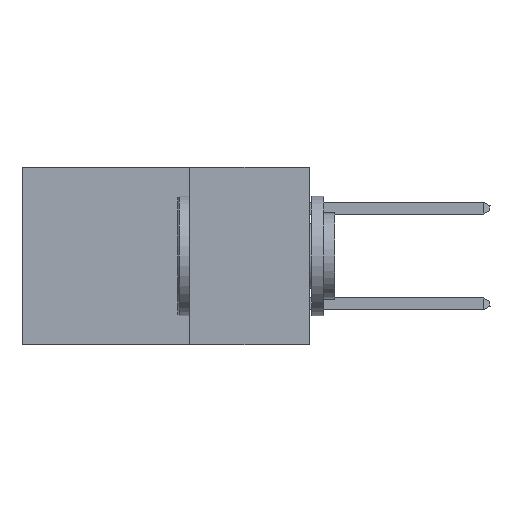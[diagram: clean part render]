
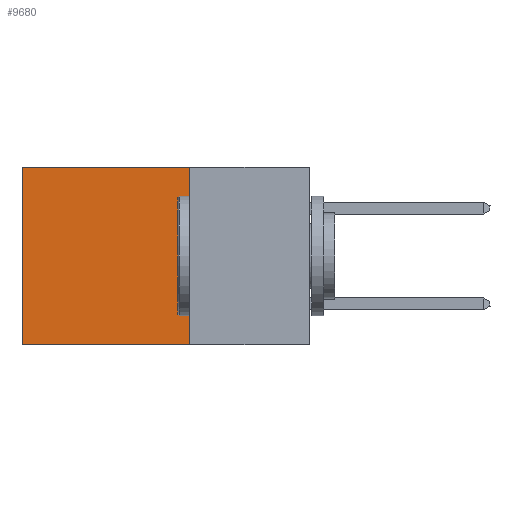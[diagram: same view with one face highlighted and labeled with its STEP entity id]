
A CAD part, left-side view. The second image highlights one B-rep face of the part: STEP entity #9680.
In plain terms, the highlighted planar face has unit normal (-1, 0, 0).
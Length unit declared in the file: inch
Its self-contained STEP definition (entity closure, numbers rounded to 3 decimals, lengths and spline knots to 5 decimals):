
#681 = DIRECTION ( 'NONE',  ( 0., 0., -1. ) ) ;
#1532 = EDGE_LOOP ( 'NONE', ( #10263, #7408, #1742, #7679 ) ) ;
#1534 = VECTOR ( 'NONE', #5011, 39.37008 ) ;
#1540 = VECTOR ( 'NONE', #8751, 39.37008 ) ;
#1742 = ORIENTED_EDGE ( 'NONE', *, *, #8023, .F. ) ;
#1813 = AXIS2_PLACEMENT_3D ( 'NONE', #2339, #5754, #681 ) ;
#1914 = CARTESIAN_POINT ( 'NONE',  ( 0.2875, 0.25, -0.37 ) ) ;
#2339 = CARTESIAN_POINT ( 'NONE',  ( 0.2875, 0.25, 0. ) ) ;
#2907 = CARTESIAN_POINT ( 'NONE',  ( 0.2875, 0.6, 0. ) ) ;
#3188 = PLANE ( 'NONE',  #1813 ) ;
#3259 = VECTOR ( 'NONE', #3657, 39.37008 ) ;
#3532 = LINE ( 'NONE', #2907, #1540 ) ;
#3657 = DIRECTION ( 'NONE',  ( 0., 1., 0. ) ) ;
#3785 = LINE ( 'NONE', #10820, #1534 ) ;
#4474 = VERTEX_POINT ( 'NONE', #10318 ) ;
#4600 = VERTEX_POINT ( 'NONE', #7164 ) ;
#4610 = CARTESIAN_POINT ( 'NONE',  ( 0.2875, 0.25, 0. ) ) ;
#5011 = DIRECTION ( 'NONE',  ( 0., 1., 0. ) ) ;
#5233 = VERTEX_POINT ( 'NONE', #7151 ) ;
#5248 = LINE ( 'NONE', #9457, #3259 ) ;
#5555 = LINE ( 'NONE', #4610, #7756 ) ;
#5754 = DIRECTION ( 'NONE',  ( 1., 0., 0. ) ) ;
#7151 = CARTESIAN_POINT ( 'NONE',  ( 0.2875, 0.25, 0. ) ) ;
#7164 = CARTESIAN_POINT ( 'NONE',  ( 0.2875, 0.6, -0.37 ) ) ;
#7372 = VERTEX_POINT ( 'NONE', #1914 ) ;
#7408 = ORIENTED_EDGE ( 'NONE', *, *, #9362, .F. ) ;
#7679 = ORIENTED_EDGE ( 'NONE', *, *, #9761, .T. ) ;
#7756 = VECTOR ( 'NONE', #8737, 39.37008 ) ;
#8023 = EDGE_CURVE ( 'NONE', #5233, #7372, #5555, .T. ) ;
#8731 = FACE_OUTER_BOUND ( 'NONE', #1532, .T. ) ;
#8737 = DIRECTION ( 'NONE',  ( 0., 0., -1. ) ) ;
#8751 = DIRECTION ( 'NONE',  ( 0., 0., -1. ) ) ;
#9362 = EDGE_CURVE ( 'NONE', #7372, #4600, #5248, .T. ) ;
#9457 = CARTESIAN_POINT ( 'NONE',  ( 0.2875, 0.25, -0.37 ) ) ;
#9680 = ADVANCED_FACE ( 'NONE', ( #8731 ), #3188, .F. ) ;
#9761 = EDGE_CURVE ( 'NONE', #5233, #4474, #3785, .T. ) ;
#10263 = ORIENTED_EDGE ( 'NONE', *, *, #10796, .T. ) ;
#10318 = CARTESIAN_POINT ( 'NONE',  ( 0.2875, 0.6, 0. ) ) ;
#10796 = EDGE_CURVE ( 'NONE', #4474, #4600, #3532, .T. ) ;
#10820 = CARTESIAN_POINT ( 'NONE',  ( 0.2875, 0.25, 0. ) ) ;
